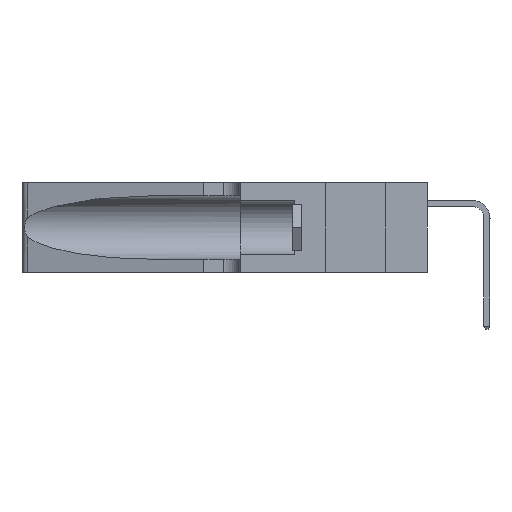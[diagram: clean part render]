
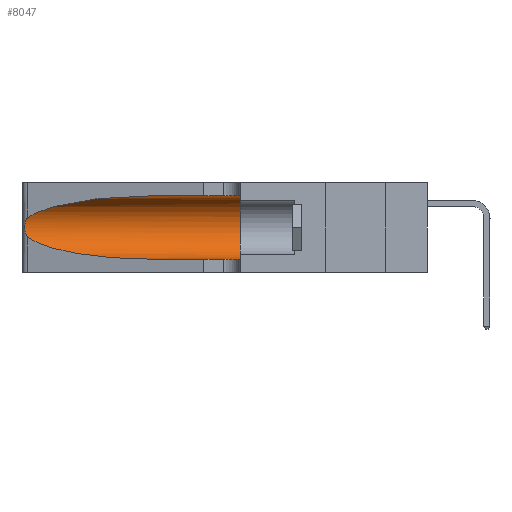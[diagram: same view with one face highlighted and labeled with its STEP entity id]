
A CAD part, left-side view. The second image highlights one B-rep face of the part: STEP entity #8047.
In plain terms, the highlighted cylindrical face has radius 3.308 mm (diameter 6.617 mm), a partial arc.
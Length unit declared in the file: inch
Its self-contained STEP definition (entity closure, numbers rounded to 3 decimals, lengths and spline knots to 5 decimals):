
#43 = CARTESIAN_POINT ( 'NONE',  ( 0.26017, 1.23833, 0.17102 ) ) ;
#144 = EDGE_CURVE ( 'NONE', #22404, #33334, #34617, .T. ) ;
#859 = CARTESIAN_POINT ( 'NONE',  ( 0.2373, 1.15595, 0.08982 ) ) ;
#1279 = LINE ( 'NONE', #23796, #8598 ) ;
#2838 = CARTESIAN_POINT ( 'NONE',  ( 0.25789, 1.23486, 0.15765 ) ) ;
#2992 =( BOUNDED_CURVE ( )  B_SPLINE_CURVE ( 3, ( #19992, #859, #6408, #25386 ),
 .UNSPECIFIED., .F., .F. ) 
 B_SPLINE_CURVE_WITH_KNOTS ( ( 4, 4 ),
 ( 3.44316, 4.71239 ),
 .UNSPECIFIED. ) 
 CURVE ( )  GEOMETRIC_REPRESENTATION_ITEM ( )  RATIONAL_B_SPLINE_CURVE ( ( 1., 0.87, 0.87, 1. ) ) 
 REPRESENTATION_ITEM ( '' )  );
#4030 = DIRECTION ( 'NONE',  ( 0., -1., 0. ) ) ;
#4182 = CARTESIAN_POINT ( 'NONE',  ( 0.2373, 1.15595, 0.28018 ) ) ;
#4547 = EDGE_CURVE ( 'NONE', #35137, #33334, #7915, .T. ) ;
#5621 = CARTESIAN_POINT ( 'NONE',  ( 0.25555, 1.22993, 0.14849 ) ) ;
#6192 = CARTESIAN_POINT ( 'NONE',  ( 0.1305, 0.72297, 0.31525 ) ) ;
#6408 = CARTESIAN_POINT ( 'NONE',  ( 0.18966, 0.96281, 0.05475 ) ) ;
#7915 = CIRCLE ( 'NONE', #28847, 0.13025 ) ;
#8047 = ADVANCED_FACE ( 'NONE', ( #17703 ), #16834, .F. ) ;
#8598 = VECTOR ( 'NONE', #18360, 39.37008 ) ;
#8655 = DIRECTION ( 'NONE',  ( 0., 1., 0. ) ) ;
#10990 = CARTESIAN_POINT ( 'NONE',  ( 0.25787, 1.23484, 0.2124 ) ) ;
#11728 = VERTEX_POINT ( 'NONE', #33006 ) ;
#13610 = CARTESIAN_POINT ( 'NONE',  ( 0.25487, 1.22718, 0.22369 ) ) ;
#13658 = DIRECTION ( 'NONE',  ( 0., -1., 0. ) ) ;
#13718 = CARTESIAN_POINT ( 'NONE',  ( 0.26018, 1.23835, 0.19895 ) ) ;
#15130 = ORIENTED_EDGE ( 'NONE', *, *, #31784, .T. ) ;
#16419 = CARTESIAN_POINT ( 'NONE',  ( 0.26075, 1.23896, 0.178 ) ) ;
#16834 = CYLINDRICAL_SURFACE ( 'NONE', #19652, 0.13025 ) ;
#17703 = FACE_OUTER_BOUND ( 'NONE', #28523, .T. ) ;
#18281 = ORIENTED_EDGE ( 'NONE', *, *, #144, .T. ) ;
#18360 = DIRECTION ( 'NONE',  ( 0., -1., 0. ) ) ;
#19180 = CARTESIAN_POINT ( 'NONE',  ( 0.25856, 1.23593, 0.16098 ) ) ;
#19302 = ORIENTED_EDGE ( 'NONE', *, *, #4547, .F. ) ;
#19615 = VERTEX_POINT ( 'NONE', #6192 ) ;
#19652 = AXIS2_PLACEMENT_3D ( 'NONE', #29856, #13658, #32580 ) ;
#19992 = CARTESIAN_POINT ( 'NONE',  ( 0.25487, 1.22718, 0.14631 ) ) ;
#20351 = CARTESIAN_POINT ( 'NONE',  ( 0.1305, 1.61858, 0.05475 ) ) ;
#20494 = CARTESIAN_POINT ( 'NONE',  ( 0.18966, 0.96281, 0.31525 ) ) ;
#21865 = ORIENTED_EDGE ( 'NONE', *, *, #26082, .T. ) ;
#21892 = CARTESIAN_POINT ( 'NONE',  ( 0.25639, 1.23186, 0.15144 ) ) ;
#22404 = VERTEX_POINT ( 'NONE', #34015 ) ;
#23205 = CARTESIAN_POINT ( 'NONE',  ( 0.25487, 1.22718, 0.22369 ) ) ;
#23796 = CARTESIAN_POINT ( 'NONE',  ( 0.1305, 1.61858, 0.31525 ) ) ;
#24535 = CARTESIAN_POINT ( 'NONE',  ( 0.25487, 1.22718, 0.22369 ) ) ;
#24586 = CARTESIAN_POINT ( 'NONE',  ( 0.25487, 1.22718, 0.14631 ) ) ;
#24888 = CARTESIAN_POINT ( 'NONE',  ( 0.1305, 0.35, 0.185 ) ) ;
#25386 = CARTESIAN_POINT ( 'NONE',  ( 0.1305, 0.72297, 0.05475 ) ) ;
#25883 = ORIENTED_EDGE ( 'NONE', *, *, #34789, .T. ) ;
#25990 = CARTESIAN_POINT ( 'NONE',  ( 0.1305, 0.35, 0.31525 ) ) ;
#26082 = EDGE_CURVE ( 'NONE', #11728, #22404, #2992, .T. ) ;
#27201 = CARTESIAN_POINT ( 'NONE',  ( 0.25639, 1.23184, 0.21858 ) ) ;
#27628 = DIRECTION ( 'NONE',  ( 0., 0., 1. ) ) ;
#28208 = EDGE_CURVE ( 'NONE', #19615, #35137, #1279, .T. ) ;
#28269 = VECTOR ( 'NONE', #4030, 39.37008 ) ;
#28392 =( BOUNDED_CURVE ( )  B_SPLINE_CURVE ( 3, ( #33966, #20494, #4182, #23205 ),
 .UNSPECIFIED., .F., .F. ) 
 B_SPLINE_CURVE_WITH_KNOTS ( ( 4, 4 ),
 ( 1.5708, 2.84003 ),
 .UNSPECIFIED. ) 
 CURVE ( )  GEOMETRIC_REPRESENTATION_ITEM ( )  RATIONAL_B_SPLINE_CURVE ( ( 1., 0.87, 0.87, 1. ) ) 
 REPRESENTATION_ITEM ( '' )  );
#28523 = EDGE_LOOP ( 'NONE', ( #15130, #25883, #21865, #18281, #19302, #35226 ) ) ;
#28847 = AXIS2_PLACEMENT_3D ( 'NONE', #24888, #8655, #27628 ) ;
#28946 = CARTESIAN_POINT ( 'NONE',  ( 0.1305, 0.35, 0.05475 ) ) ;
#29016 = VERTEX_POINT ( 'NONE', #24535 ) ;
#29800 = CARTESIAN_POINT ( 'NONE',  ( 0.25555, 1.22994, 0.2215 ) ) ;
#29856 = CARTESIAN_POINT ( 'NONE',  ( 0.1305, 1.61858, 0.185 ) ) ;
#29926 = CARTESIAN_POINT ( 'NONE',  ( 0.25854, 1.2359, 0.20912 ) ) ;
#31784 = EDGE_CURVE ( 'NONE', #19615, #29016, #28392, .T. ) ;
#32580 = DIRECTION ( 'NONE',  ( 0., 0., -1. ) ) ;
#32653 = CARTESIAN_POINT ( 'NONE',  ( 0.26075, 1.23896, 0.19203 ) ) ;
#33006 = CARTESIAN_POINT ( 'NONE',  ( 0.25487, 1.22718, 0.14631 ) ) ;
#33334 = VERTEX_POINT ( 'NONE', #28946 ) ;
#33397 = B_SPLINE_CURVE_WITH_KNOTS ( 'NONE', 3,
 ( #13610, #29800, #27201, #10990, #29926, #13718, #32653, #16419, #43, #19180, #2838, #21892, #5621, #24586 ),
 .UNSPECIFIED., .F., .F.,
 ( 4, 2, 2, 2, 2, 2, 4 ),
 ( 0., 0.00027, 0.00053, 0.00107, 0.0016, 0.00187, 0.00214 ),
 .UNSPECIFIED. ) ;
#33966 = CARTESIAN_POINT ( 'NONE',  ( 0.1305, 0.72297, 0.31525 ) ) ;
#34015 = CARTESIAN_POINT ( 'NONE',  ( 0.1305, 0.72297, 0.05475 ) ) ;
#34617 = LINE ( 'NONE', #20351, #28269 ) ;
#34789 = EDGE_CURVE ( 'NONE', #29016, #11728, #33397, .T. ) ;
#35137 = VERTEX_POINT ( 'NONE', #25990 ) ;
#35226 = ORIENTED_EDGE ( 'NONE', *, *, #28208, .F. ) ;
